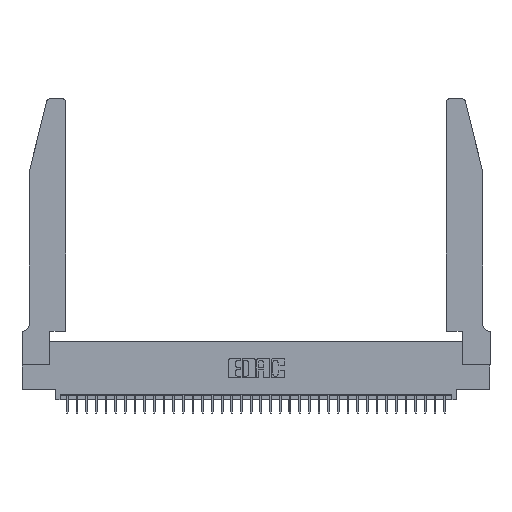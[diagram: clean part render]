
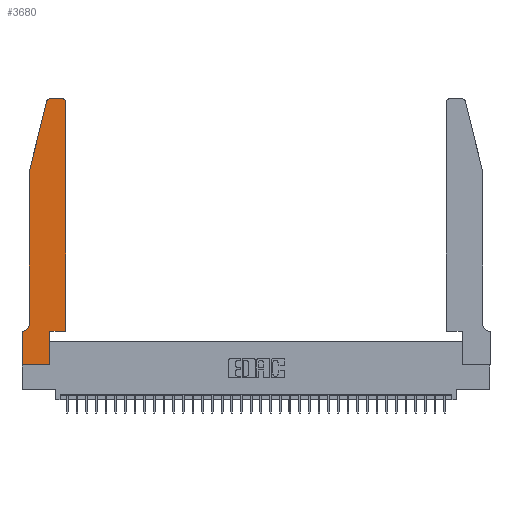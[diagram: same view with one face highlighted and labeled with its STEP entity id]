
A CAD part, top view. The second image highlights one B-rep face of the part: STEP entity #3680.
In plain terms, the highlighted planar face has unit normal (0, 0, 1).
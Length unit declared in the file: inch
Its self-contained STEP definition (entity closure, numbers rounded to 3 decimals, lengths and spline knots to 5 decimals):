
#579 = EDGE_CURVE ( 'NONE', #11929, #3285, #15734, .T. ) ;
#911 = VECTOR ( 'NONE', #1713, 39.37008 ) ;
#1154 = DIRECTION ( 'NONE',  ( 1., 0., 0. ) ) ;
#1386 = VECTOR ( 'NONE', #21525, 39.37008 ) ;
#1507 = CARTESIAN_POINT ( 'NONE',  ( 0.284, 2.75, 0.37 ) ) ;
#1707 = ORIENTED_EDGE ( 'NONE', *, *, #3159, .T. ) ;
#1713 = DIRECTION ( 'NONE',  ( 0., 1., 0. ) ) ;
#1755 = LINE ( 'NONE', #24315, #1386 ) ;
#2189 = LINE ( 'NONE', #33537, #7764 ) ;
#3159 = EDGE_CURVE ( 'NONE', #14699, #11951, #2189, .T. ) ;
#3242 = ORIENTED_EDGE ( 'NONE', *, *, #579, .T. ) ;
#3285 = VERTEX_POINT ( 'NONE', #13376 ) ;
#3455 = ORIENTED_EDGE ( 'NONE', *, *, #28499, .T. ) ;
#3530 = VERTEX_POINT ( 'NONE', #35240 ) ;
#3680 = ADVANCED_FACE ( 'NONE', ( #28915 ), #34498, .T. ) ;
#4697 = CARTESIAN_POINT ( 'NONE',  ( 0.0055, 0.42, 0.37 ) ) ;
#5497 = DIRECTION ( 'NONE',  ( 1., 0., 0. ) ) ;
#6486 = CARTESIAN_POINT ( 'NONE',  ( 0., 0.35, 0.37 ) ) ;
#7385 = EDGE_CURVE ( 'NONE', #3530, #15056, #1755, .T. ) ;
#7420 = CARTESIAN_POINT ( 'NONE',  ( 0., 0., 0.37 ) ) ;
#7764 = VECTOR ( 'NONE', #36641, 39.37008 ) ;
#8292 = CARTESIAN_POINT ( 'NONE',  ( 0., 0., 0.37 ) ) ;
#8536 = CIRCLE ( 'NONE', #29845, 0.03 ) ;
#9033 = ORIENTED_EDGE ( 'NONE', *, *, #10714, .T. ) ;
#9662 = EDGE_CURVE ( 'NONE', #3285, #14699, #34350, .T. ) ;
#9843 = CARTESIAN_POINT ( 'NONE',  ( 0.2865, 0.35, 0.37 ) ) ;
#10037 = DIRECTION ( 'NONE',  ( 0., 0., -1. ) ) ;
#10216 = DIRECTION ( 'NONE',  ( -1., 0., 0. ) ) ;
#10639 = VECTOR ( 'NONE', #25751, 39.37008 ) ;
#10714 = EDGE_CURVE ( 'NONE', #11507, #33598, #11089, .T. ) ;
#11089 = LINE ( 'NONE', #22410, #10639 ) ;
#11195 = AXIS2_PLACEMENT_3D ( 'NONE', #29210, #29962, #12322 ) ;
#11507 = VERTEX_POINT ( 'NONE', #29960 ) ;
#11929 = VERTEX_POINT ( 'NONE', #29298 ) ;
#11951 = VERTEX_POINT ( 'NONE', #1507 ) ;
#12322 = DIRECTION ( 'NONE',  ( 1., 0., 0. ) ) ;
#12504 = VERTEX_POINT ( 'NONE', #33917 ) ;
#13346 = AXIS2_PLACEMENT_3D ( 'NONE', #4697, #10037, #10216 ) ;
#13376 = CARTESIAN_POINT ( 'NONE',  ( 0.4505, 2.72, 0.37 ) ) ;
#13452 = ORIENTED_EDGE ( 'NONE', *, *, #28474, .T. ) ;
#13559 = EDGE_CURVE ( 'NONE', #33598, #3530, #26999, .T. ) ;
#14029 = VERTEX_POINT ( 'NONE', #7420 ) ;
#14699 = VERTEX_POINT ( 'NONE', #23924 ) ;
#14875 = EDGE_LOOP ( 'NONE', ( #1707, #32094, #3455, #9033, #18937, #30290, #16879, #13452, #22738, #19269, #3242, #27649 ) ) ;
#15023 = EDGE_CURVE ( 'NONE', #31807, #11929, #21809, .T. ) ;
#15056 = VERTEX_POINT ( 'NONE', #25147 ) ;
#15208 = CARTESIAN_POINT ( 'NONE',  ( 0., 0., 0.37 ) ) ;
#15734 = LINE ( 'NONE', #27085, #911 ) ;
#16879 = ORIENTED_EDGE ( 'NONE', *, *, #35422, .T. ) ;
#17186 = CARTESIAN_POINT ( 'NONE',  ( 0.284, 2.72, 0.37 ) ) ;
#18478 = CARTESIAN_POINT ( 'NONE',  ( 0.2865, 0.35, 0.37 ) ) ;
#18937 = ORIENTED_EDGE ( 'NONE', *, *, #13559, .T. ) ;
#19269 = ORIENTED_EDGE ( 'NONE', *, *, #15023, .T. ) ;
#19563 = DIRECTION ( 'NONE',  ( 0., -1., 0. ) ) ;
#19991 = CARTESIAN_POINT ( 'NONE',  ( 0.25487, 2.72718, 0.37 ) ) ;
#20428 = LINE ( 'NONE', #15208, #35932 ) ;
#20614 = DIRECTION ( 'NONE',  ( -0.239, -0.971, 0. ) ) ;
#20810 = VERTEX_POINT ( 'NONE', #19991 ) ;
#20965 = CARTESIAN_POINT ( 'NONE',  ( 0.0755, 2., 0.37 ) ) ;
#21525 = DIRECTION ( 'NONE',  ( -1., 0., 0. ) ) ;
#21809 = LINE ( 'NONE', #31109, #23531 ) ;
#22410 = CARTESIAN_POINT ( 'NONE',  ( 0.0755, 2., 0.37 ) ) ;
#22738 = ORIENTED_EDGE ( 'NONE', *, *, #29612, .T. ) ;
#23531 = VECTOR ( 'NONE', #5497, 39.37008 ) ;
#23675 = EDGE_CURVE ( 'NONE', #11951, #20810, #8536, .T. ) ;
#23924 = CARTESIAN_POINT ( 'NONE',  ( 0.4205, 2.75, 0.37 ) ) ;
#24315 = CARTESIAN_POINT ( 'NONE',  ( 0.0755, 0.35, 0.37 ) ) ;
#24812 = CARTESIAN_POINT ( 'NONE',  ( 0.0755, 0.42, 0.37 ) ) ;
#24945 = AXIS2_PLACEMENT_3D ( 'NONE', #6486, #28737, #31913 ) ;
#25147 = CARTESIAN_POINT ( 'NONE',  ( 0., 0.35, 0.37 ) ) ;
#25179 = DIRECTION ( 'NONE',  ( 0., 0., 1. ) ) ;
#25376 = DIRECTION ( 'NONE',  ( 1., 0., 0. ) ) ;
#25751 = DIRECTION ( 'NONE',  ( 0., -1., 0. ) ) ;
#26174 = LINE ( 'NONE', #20965, #34184 ) ;
#26999 = CIRCLE ( 'NONE', #13346, 0.07 ) ;
#27081 = VECTOR ( 'NONE', #32848, 39.37008 ) ;
#27085 = CARTESIAN_POINT ( 'NONE',  ( 0.4505, 0.35, 0.37 ) ) ;
#27649 = ORIENTED_EDGE ( 'NONE', *, *, #9662, .T. ) ;
#28474 = EDGE_CURVE ( 'NONE', #14029, #12504, #20428, .T. ) ;
#28499 = EDGE_CURVE ( 'NONE', #20810, #11507, #26174, .T. ) ;
#28737 = DIRECTION ( 'NONE',  ( 0., 0., 1. ) ) ;
#28915 = FACE_OUTER_BOUND ( 'NONE', #14875, .T. ) ;
#29210 = CARTESIAN_POINT ( 'NONE',  ( 0.4205, 2.72, 0.37 ) ) ;
#29298 = CARTESIAN_POINT ( 'NONE',  ( 0.4505, 0.35, 0.37 ) ) ;
#29612 = EDGE_CURVE ( 'NONE', #12504, #31807, #30031, .T. ) ;
#29845 = AXIS2_PLACEMENT_3D ( 'NONE', #17186, #25179, #25376 ) ;
#29960 = CARTESIAN_POINT ( 'NONE',  ( 0.0755, 2., 0.37 ) ) ;
#29962 = DIRECTION ( 'NONE',  ( 0., 0., 1. ) ) ;
#30031 = LINE ( 'NONE', #18478, #27081 ) ;
#30290 = ORIENTED_EDGE ( 'NONE', *, *, #7385, .T. ) ;
#31109 = CARTESIAN_POINT ( 'NONE',  ( 0.4505, 0.35, 0.37 ) ) ;
#31807 = VERTEX_POINT ( 'NONE', #9843 ) ;
#31913 = DIRECTION ( 'NONE',  ( 1., 0., 0. ) ) ;
#32094 = ORIENTED_EDGE ( 'NONE', *, *, #23675, .T. ) ;
#32848 = DIRECTION ( 'NONE',  ( 0., 1., 0. ) ) ;
#33537 = CARTESIAN_POINT ( 'NONE',  ( 0.2605, 2.75, 0.37 ) ) ;
#33598 = VERTEX_POINT ( 'NONE', #24812 ) ;
#33757 = LINE ( 'NONE', #8292, #36376 ) ;
#33917 = CARTESIAN_POINT ( 'NONE',  ( 0.2865, 0., 0.37 ) ) ;
#34184 = VECTOR ( 'NONE', #20614, 39.37008 ) ;
#34350 = CIRCLE ( 'NONE', #11195, 0.03 ) ;
#34498 = PLANE ( 'NONE',  #24945 ) ;
#35240 = CARTESIAN_POINT ( 'NONE',  ( 0.0055, 0.35, 0.37 ) ) ;
#35422 = EDGE_CURVE ( 'NONE', #15056, #14029, #33757, .T. ) ;
#35932 = VECTOR ( 'NONE', #1154, 39.37008 ) ;
#36376 = VECTOR ( 'NONE', #19563, 39.37008 ) ;
#36641 = DIRECTION ( 'NONE',  ( -1., 0., 0. ) ) ;
